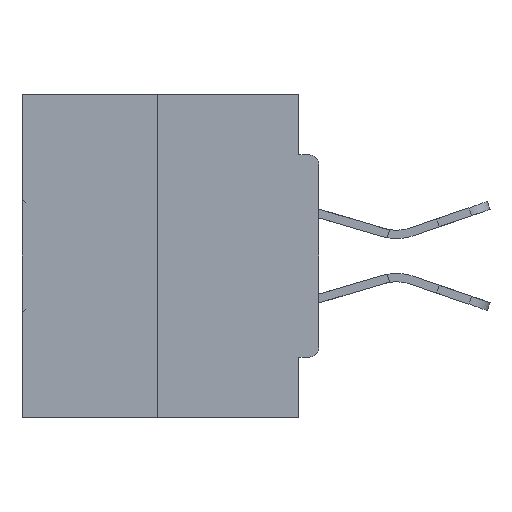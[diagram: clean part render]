
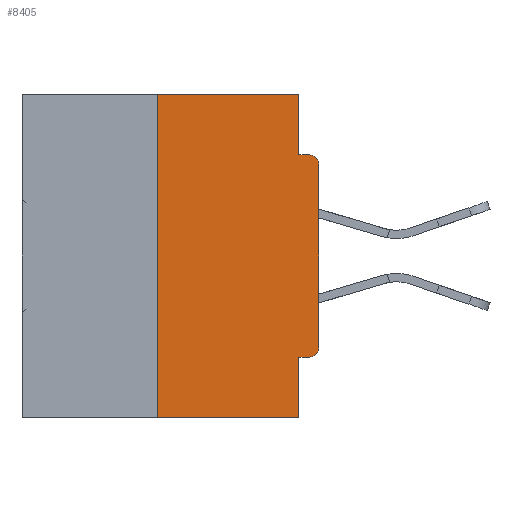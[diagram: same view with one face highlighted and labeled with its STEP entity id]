
A CAD part, left-side view. The second image highlights one B-rep face of the part: STEP entity #8405.
In plain terms, the highlighted planar face has unit normal (-1, 0, 0).
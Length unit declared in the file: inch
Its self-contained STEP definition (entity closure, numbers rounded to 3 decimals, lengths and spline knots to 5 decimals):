
#877 = LINE ( 'NONE', #35900, #18370 ) ;
#1014 = CARTESIAN_POINT ( 'NONE',  ( 0., 0., -0.1085 ) ) ;
#1277 = CARTESIAN_POINT ( 'NONE',  ( 0., 0.031, 0. ) ) ;
#1898 = ORIENTED_EDGE ( 'NONE', *, *, #12098, .F. ) ;
#2122 = LINE ( 'NONE', #34483, #32697 ) ;
#2163 = DIRECTION ( 'NONE',  ( 0., 0., -1. ) ) ;
#2382 = ORIENTED_EDGE ( 'NONE', *, *, #35666, .F. ) ;
#3378 = VERTEX_POINT ( 'NONE', #1014 ) ;
#5299 = LINE ( 'NONE', #26984, #7448 ) ;
#5339 = CARTESIAN_POINT ( 'NONE',  ( 0., 0.031, -0.0935 ) ) ;
#5342 = VERTEX_POINT ( 'NONE', #19006 ) ;
#6596 = VERTEX_POINT ( 'NONE', #40459 ) ;
#7448 = VECTOR ( 'NONE', #23775, 39.37008 ) ;
#7817 = CARTESIAN_POINT ( 'NONE',  ( 0., 0., -0.3915 ) ) ;
#7912 = EDGE_CURVE ( 'NONE', #33251, #41374, #33791, .T. ) ;
#8028 = ORIENTED_EDGE ( 'NONE', *, *, #7912, .F. ) ;
#8173 = CARTESIAN_POINT ( 'NONE',  ( 0., 0.031, -0.4065 ) ) ;
#8337 = CARTESIAN_POINT ( 'NONE',  ( 0., 0.25, 0. ) ) ;
#8405 = ADVANCED_FACE ( 'NONE', ( #11619 ), #22411, .F. ) ;
#9013 = DIRECTION ( 'NONE',  ( -1., 0., 0. ) ) ;
#9235 = DIRECTION ( 'NONE',  ( 0., 0., 1. ) ) ;
#10148 = EDGE_CURVE ( 'NONE', #39612, #5342, #2122, .T. ) ;
#11619 = FACE_OUTER_BOUND ( 'NONE', #21789, .T. ) ;
#11760 = ORIENTED_EDGE ( 'NONE', *, *, #18133, .F. ) ;
#12098 = EDGE_CURVE ( 'NONE', #29258, #12642, #33033, .T. ) ;
#12339 = DIRECTION ( 'NONE',  ( 0., 1., 0. ) ) ;
#12642 = VERTEX_POINT ( 'NONE', #13962 ) ;
#12909 = VERTEX_POINT ( 'NONE', #5339 ) ;
#13079 = EDGE_CURVE ( 'NONE', #33251, #27037, #31916, .T. ) ;
#13962 = CARTESIAN_POINT ( 'NONE',  ( 0., 0.031, 0. ) ) ;
#14340 = DIRECTION ( 'NONE',  ( 0., -1., 0. ) ) ;
#15095 = AXIS2_PLACEMENT_3D ( 'NONE', #19294, #25816, #2163 ) ;
#16397 = DIRECTION ( 'NONE',  ( 0., -1., 0. ) ) ;
#17517 = VECTOR ( 'NONE', #12339, 39.37008 ) ;
#17897 = ORIENTED_EDGE ( 'NONE', *, *, #13079, .T. ) ;
#18133 = EDGE_CURVE ( 'NONE', #41374, #5342, #42176, .T. ) ;
#18217 = ORIENTED_EDGE ( 'NONE', *, *, #32000, .T. ) ;
#18370 = VECTOR ( 'NONE', #9235, 39.37008 ) ;
#18706 = CARTESIAN_POINT ( 'NONE',  ( 0., 0.031, -0.5 ) ) ;
#18998 = CARTESIAN_POINT ( 'NONE',  ( 0., 0., -0.0935 ) ) ;
#19006 = CARTESIAN_POINT ( 'NONE',  ( 0., 0.031, -0.5 ) ) ;
#19226 = DIRECTION ( 'NONE',  ( 0., 0., -1. ) ) ;
#19294 = CARTESIAN_POINT ( 'NONE',  ( 0., 0.46, 0. ) ) ;
#20392 = VECTOR ( 'NONE', #36028, 39.37008 ) ;
#20462 = ORIENTED_EDGE ( 'NONE', *, *, #42291, .F. ) ;
#20463 = CARTESIAN_POINT ( 'NONE',  ( 0., 0.015, -0.4065 ) ) ;
#21789 = EDGE_LOOP ( 'NONE', ( #1898, #2382, #31655, #11760, #8028, #17897, #39751, #18217, #20462, #29907 ) ) ;
#22411 = PLANE ( 'NONE',  #15095 ) ;
#23775 = DIRECTION ( 'NONE',  ( 0., 0., 1. ) ) ;
#24145 = EDGE_CURVE ( 'NONE', #12642, #12909, #33399, .T. ) ;
#24399 = VECTOR ( 'NONE', #32343, 39.37008 ) ;
#25192 = CARTESIAN_POINT ( 'NONE',  ( 0., 0.015, -0.1085 ) ) ;
#25816 = DIRECTION ( 'NONE',  ( 1., 0., 0. ) ) ;
#26984 = CARTESIAN_POINT ( 'NONE',  ( 0., 0.25, 0. ) ) ;
#27037 = VERTEX_POINT ( 'NONE', #7817 ) ;
#29253 = CARTESIAN_POINT ( 'NONE',  ( 0., 0.015, -0.3915 ) ) ;
#29258 = VERTEX_POINT ( 'NONE', #8337 ) ;
#29907 = ORIENTED_EDGE ( 'NONE', *, *, #24145, .F. ) ;
#30421 = VECTOR ( 'NONE', #16397, 39.37008 ) ;
#31349 = VECTOR ( 'NONE', #38782, 39.37008 ) ;
#31655 = ORIENTED_EDGE ( 'NONE', *, *, #10148, .T. ) ;
#31916 = CIRCLE ( 'NONE', #37142, 0.015 ) ;
#32000 = EDGE_CURVE ( 'NONE', #3378, #6596, #32579, .T. ) ;
#32343 = DIRECTION ( 'NONE',  ( 0., 0., -1. ) ) ;
#32579 = CIRCLE ( 'NONE', #38363, 0.015 ) ;
#32602 = DIRECTION ( 'NONE',  ( 0., 0., -1. ) ) ;
#32697 = VECTOR ( 'NONE', #14340, 39.37008 ) ;
#33033 = LINE ( 'NONE', #43566, #30421 ) ;
#33251 = VERTEX_POINT ( 'NONE', #20463 ) ;
#33399 = LINE ( 'NONE', #1277, #31349 ) ;
#33791 = LINE ( 'NONE', #42234, #17517 ) ;
#34483 = CARTESIAN_POINT ( 'NONE',  ( 0., 0.46, -0.5 ) ) ;
#35666 = EDGE_CURVE ( 'NONE', #39612, #29258, #5299, .T. ) ;
#35900 = CARTESIAN_POINT ( 'NONE',  ( 0., 0., 0. ) ) ;
#36028 = DIRECTION ( 'NONE',  ( 0., -1., 0. ) ) ;
#37142 = AXIS2_PLACEMENT_3D ( 'NONE', #29253, #9013, #19226 ) ;
#37736 = EDGE_CURVE ( 'NONE', #27037, #3378, #877, .T. ) ;
#38363 = AXIS2_PLACEMENT_3D ( 'NONE', #25192, #43153, #32602 ) ;
#38501 = CARTESIAN_POINT ( 'NONE',  ( 0., 0.25, -0.5 ) ) ;
#38782 = DIRECTION ( 'NONE',  ( 0., 0., -1. ) ) ;
#39612 = VERTEX_POINT ( 'NONE', #38501 ) ;
#39751 = ORIENTED_EDGE ( 'NONE', *, *, #37736, .T. ) ;
#40459 = CARTESIAN_POINT ( 'NONE',  ( 0., 0.015, -0.0935 ) ) ;
#41374 = VERTEX_POINT ( 'NONE', #8173 ) ;
#42176 = LINE ( 'NONE', #18706, #24399 ) ;
#42234 = CARTESIAN_POINT ( 'NONE',  ( 0., 0., -0.4065 ) ) ;
#42291 = EDGE_CURVE ( 'NONE', #12909, #6596, #43464, .T. ) ;
#43153 = DIRECTION ( 'NONE',  ( -1., 0., 0. ) ) ;
#43464 = LINE ( 'NONE', #18998, #20392 ) ;
#43566 = CARTESIAN_POINT ( 'NONE',  ( 0., 0.46, 0. ) ) ;
